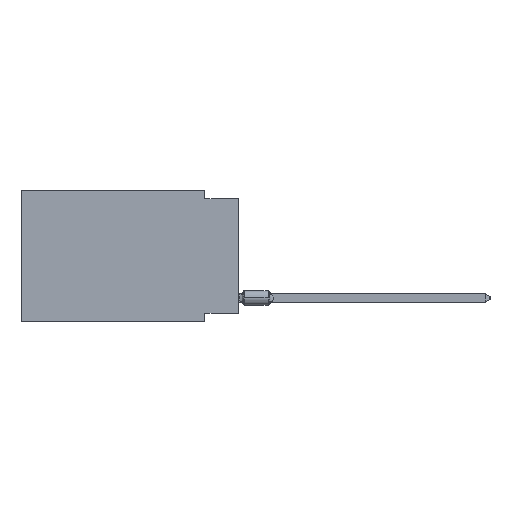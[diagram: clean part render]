
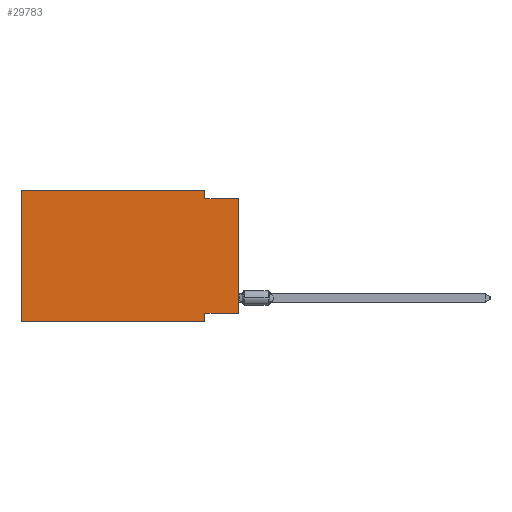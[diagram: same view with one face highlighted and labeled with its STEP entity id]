
A CAD part, left-side view. The second image highlights one B-rep face of the part: STEP entity #29783.
In plain terms, the highlighted planar face has unit normal (-1, 0, 0).
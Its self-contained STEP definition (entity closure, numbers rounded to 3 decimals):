
#379 = DIRECTION ( 'NONE',  ( 0., -1., 0. ) ) ;
#902 = CARTESIAN_POINT ( 'NONE',  ( 0., 2.54, -9.906 ) ) ;
#1143 = DIRECTION ( 'NONE',  ( 0., 0., -1. ) ) ;
#2608 = CARTESIAN_POINT ( 'NONE',  ( 0., 0., -9.271 ) ) ;
#2703 = CARTESIAN_POINT ( 'NONE',  ( 0., 0., -0.635 ) ) ;
#3403 = VERTEX_POINT ( 'NONE', #47614 ) ;
#3669 = CARTESIAN_POINT ( 'NONE',  ( 0., 0., -9.271 ) ) ;
#3866 = EDGE_CURVE ( 'NONE', #9761, #19363, #11871, .T. ) ;
#3939 = DIRECTION ( 'NONE',  ( 1., 0., 0. ) ) ;
#4029 = DIRECTION ( 'NONE',  ( 0., 0., 1. ) ) ;
#4983 = LINE ( 'NONE', #15289, #37267 ) ;
#5064 = EDGE_CURVE ( 'NONE', #28909, #23743, #11638, .T. ) ;
#6015 = EDGE_CURVE ( 'NONE', #37565, #17862, #36147, .T. ) ;
#6924 = ORIENTED_EDGE ( 'NONE', *, *, #3866, .T. ) ;
#7111 = DIRECTION ( 'NONE',  ( 0., 0., -1. ) ) ;
#8367 = EDGE_CURVE ( 'NONE', #17862, #19363, #37643, .T. ) ;
#9761 = VERTEX_POINT ( 'NONE', #36600 ) ;
#10239 = VECTOR ( 'NONE', #23869, 1000. ) ;
#11638 = LINE ( 'NONE', #26826, #10239 ) ;
#11871 = LINE ( 'NONE', #37843, #29775 ) ;
#12269 = DIRECTION ( 'NONE',  ( 0., 0., -1. ) ) ;
#12796 = DIRECTION ( 'NONE',  ( 0., -1., 0. ) ) ;
#15183 = DIRECTION ( 'NONE',  ( 0., 0., 1. ) ) ;
#15289 = CARTESIAN_POINT ( 'NONE',  ( 0., 0., 0. ) ) ;
#16731 = ORIENTED_EDGE ( 'NONE', *, *, #47276, .F. ) ;
#17401 = VECTOR ( 'NONE', #17548, 1000. ) ;
#17548 = DIRECTION ( 'NONE',  ( 0., 1., 0. ) ) ;
#17862 = VERTEX_POINT ( 'NONE', #21282 ) ;
#18295 = CARTESIAN_POINT ( 'NONE',  ( 0., 16.383, 0. ) ) ;
#18633 = PLANE ( 'NONE',  #37989 ) ;
#19363 = VERTEX_POINT ( 'NONE', #38433 ) ;
#20392 = LINE ( 'NONE', #46342, #35595 ) ;
#20736 = VECTOR ( 'NONE', #12269, 1000. ) ;
#21282 = CARTESIAN_POINT ( 'NONE',  ( 0., 2.54, -9.271 ) ) ;
#22432 = ORIENTED_EDGE ( 'NONE', *, *, #6015, .F. ) ;
#22734 = VECTOR ( 'NONE', #1143, 1000. ) ;
#22802 = CARTESIAN_POINT ( 'NONE',  ( 0., 16.383, 0. ) ) ;
#23247 = ORIENTED_EDGE ( 'NONE', *, *, #5064, .F. ) ;
#23352 = ORIENTED_EDGE ( 'NONE', *, *, #8367, .F. ) ;
#23743 = VERTEX_POINT ( 'NONE', #2703 ) ;
#23869 = DIRECTION ( 'NONE',  ( 0., -1., 0. ) ) ;
#24515 = CARTESIAN_POINT ( 'NONE',  ( 0., 16.383, 0. ) ) ;
#24772 = EDGE_LOOP ( 'NONE', ( #26948, #23247, #41115, #43144, #16731, #6924, #23352, #22432 ) ) ;
#26467 = FACE_OUTER_BOUND ( 'NONE', #24772, .T. ) ;
#26826 = CARTESIAN_POINT ( 'NONE',  ( 0., 0., -0.635 ) ) ;
#26948 = ORIENTED_EDGE ( 'NONE', *, *, #35687, .T. ) ;
#28909 = VERTEX_POINT ( 'NONE', #46747 ) ;
#29519 = EDGE_CURVE ( 'NONE', #46502, #3403, #20392, .T. ) ;
#29775 = VECTOR ( 'NONE', #379, 1000. ) ;
#29783 = ADVANCED_FACE ( 'NONE', ( #26467 ), #18633, .F. ) ;
#32551 = LINE ( 'NONE', #24515, #40999 ) ;
#34943 = EDGE_CURVE ( 'NONE', #3403, #28909, #38721, .T. ) ;
#35595 = VECTOR ( 'NONE', #12796, 1000. ) ;
#35687 = EDGE_CURVE ( 'NONE', #37565, #23743, #4983, .T. ) ;
#36147 = LINE ( 'NONE', #2608, #17401 ) ;
#36600 = CARTESIAN_POINT ( 'NONE',  ( 0., 16.383, -9.906 ) ) ;
#37267 = VECTOR ( 'NONE', #4029, 1000. ) ;
#37565 = VERTEX_POINT ( 'NONE', #3669 ) ;
#37643 = LINE ( 'NONE', #902, #22734 ) ;
#37843 = CARTESIAN_POINT ( 'NONE',  ( 0., 16.383, -9.906 ) ) ;
#37989 = AXIS2_PLACEMENT_3D ( 'NONE', #22802, #3939, #7111 ) ;
#38433 = CARTESIAN_POINT ( 'NONE',  ( 0., 2.54, -9.906 ) ) ;
#38721 = LINE ( 'NONE', #46305, #20736 ) ;
#40999 = VECTOR ( 'NONE', #15183, 1000. ) ;
#41115 = ORIENTED_EDGE ( 'NONE', *, *, #34943, .F. ) ;
#43144 = ORIENTED_EDGE ( 'NONE', *, *, #29519, .F. ) ;
#46305 = CARTESIAN_POINT ( 'NONE',  ( 0., 2.54, 0. ) ) ;
#46342 = CARTESIAN_POINT ( 'NONE',  ( 0., 16.383, 0. ) ) ;
#46502 = VERTEX_POINT ( 'NONE', #18295 ) ;
#46747 = CARTESIAN_POINT ( 'NONE',  ( 0., 2.54, -0.635 ) ) ;
#47276 = EDGE_CURVE ( 'NONE', #9761, #46502, #32551, .T. ) ;
#47614 = CARTESIAN_POINT ( 'NONE',  ( 0., 2.54, 0. ) ) ;
